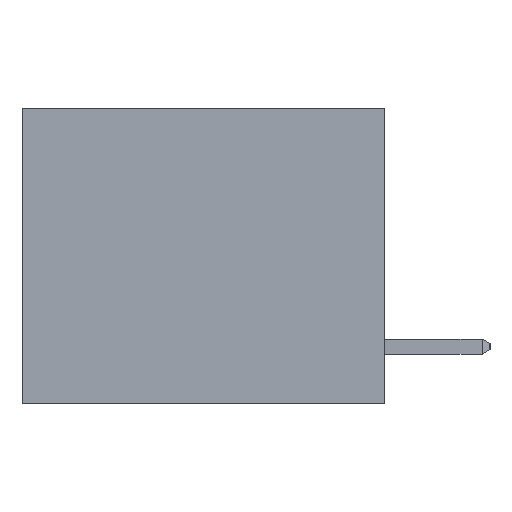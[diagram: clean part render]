
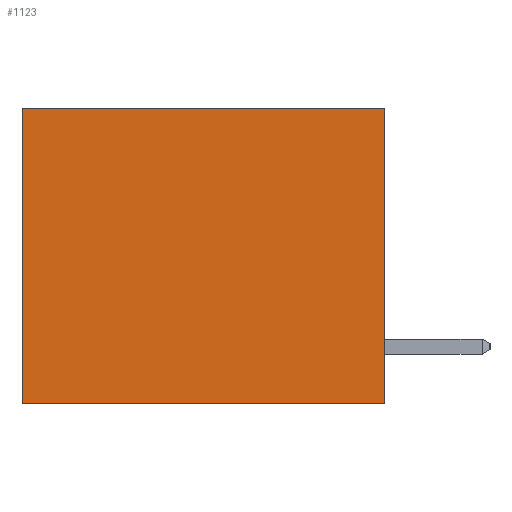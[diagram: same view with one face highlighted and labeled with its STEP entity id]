
A CAD part, left-side view. The second image highlights one B-rep face of the part: STEP entity #1123.
In plain terms, the highlighted planar face has unit normal (-1, 0, 0).
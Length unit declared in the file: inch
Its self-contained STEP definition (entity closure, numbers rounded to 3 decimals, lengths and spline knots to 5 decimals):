
#495 = LINE ( 'NONE', #4347, #10058 ) ;
#543 = ORIENTED_EDGE ( 'NONE', *, *, #20092, .F. ) ;
#1057 = FACE_OUTER_BOUND ( 'NONE', #18559, .T. ) ;
#1123 = ADVANCED_FACE ( 'NONE', ( #1057 ), #9416, .F. ) ;
#1727 = CARTESIAN_POINT ( 'NONE',  ( 0.3165, 0., 0. ) ) ;
#2391 = VERTEX_POINT ( 'NONE', #1727 ) ;
#2466 = EDGE_CURVE ( 'NONE', #2391, #18212, #22287, .T. ) ;
#2468 = LINE ( 'NONE', #4484, #13466 ) ;
#2912 = VECTOR ( 'NONE', #16324, 39.37008 ) ;
#2974 = ORIENTED_EDGE ( 'NONE', *, *, #2466, .T. ) ;
#3703 = CARTESIAN_POINT ( 'NONE',  ( 0.3165, 0., 0. ) ) ;
#4347 = CARTESIAN_POINT ( 'NONE',  ( 0.3165, 0.6, -0.49 ) ) ;
#4484 = CARTESIAN_POINT ( 'NONE',  ( 0.3165, 0., -0.49 ) ) ;
#5774 = DIRECTION ( 'NONE',  ( 1., 0., 0. ) ) ;
#7855 = LINE ( 'NONE', #10719, #2912 ) ;
#8008 = CARTESIAN_POINT ( 'NONE',  ( 0.3165, 0.6, -0.49 ) ) ;
#9416 = PLANE ( 'NONE',  #22005 ) ;
#10058 = VECTOR ( 'NONE', #19066, 39.37008 ) ;
#10719 = CARTESIAN_POINT ( 'NONE',  ( 0.3165, 0., -0.49 ) ) ;
#11314 = VECTOR ( 'NONE', #23654, 39.37008 ) ;
#12663 = EDGE_CURVE ( 'NONE', #18212, #13714, #495, .T. ) ;
#13406 = DIRECTION ( 'NONE',  ( 0., 0., -1. ) ) ;
#13466 = VECTOR ( 'NONE', #17441, 39.37008 ) ;
#13714 = VERTEX_POINT ( 'NONE', #8008 ) ;
#14741 = CARTESIAN_POINT ( 'NONE',  ( 0.3165, 0.6, 0. ) ) ;
#14935 = VERTEX_POINT ( 'NONE', #21980 ) ;
#15012 = EDGE_CURVE ( 'NONE', #14935, #13714, #2468, .T. ) ;
#16324 = DIRECTION ( 'NONE',  ( 0., 0., -1. ) ) ;
#17062 = ORIENTED_EDGE ( 'NONE', *, *, #15012, .F. ) ;
#17441 = DIRECTION ( 'NONE',  ( 0., 1., 0. ) ) ;
#18212 = VERTEX_POINT ( 'NONE', #14741 ) ;
#18559 = EDGE_LOOP ( 'NONE', ( #20793, #17062, #543, #2974 ) ) ;
#18960 = CARTESIAN_POINT ( 'NONE',  ( 0.3165, 0., -0.49 ) ) ;
#19066 = DIRECTION ( 'NONE',  ( 0., 0., -1. ) ) ;
#20092 = EDGE_CURVE ( 'NONE', #2391, #14935, #7855, .T. ) ;
#20793 = ORIENTED_EDGE ( 'NONE', *, *, #12663, .T. ) ;
#21980 = CARTESIAN_POINT ( 'NONE',  ( 0.3165, 0., -0.49 ) ) ;
#22005 = AXIS2_PLACEMENT_3D ( 'NONE', #18960, #5774, #13406 ) ;
#22287 = LINE ( 'NONE', #3703, #11314 ) ;
#23654 = DIRECTION ( 'NONE',  ( 0., 1., 0. ) ) ;
